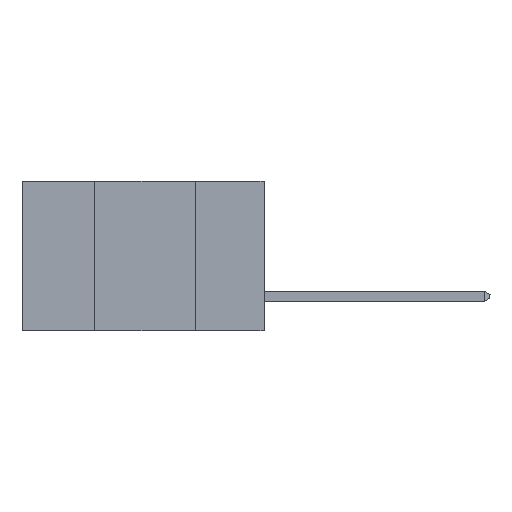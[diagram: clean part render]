
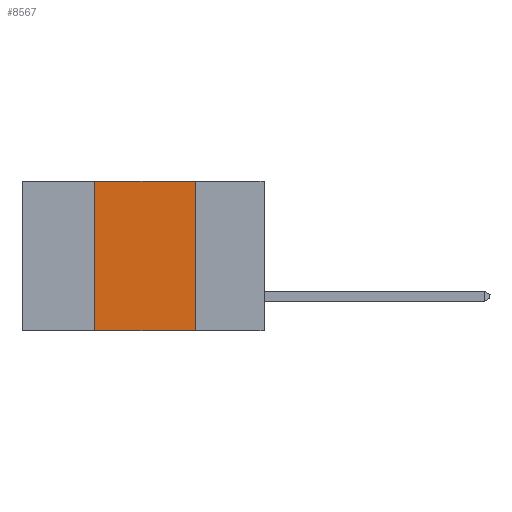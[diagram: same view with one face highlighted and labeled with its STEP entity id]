
A CAD part, left-side view. The second image highlights one B-rep face of the part: STEP entity #8567.
In plain terms, the highlighted planar face has unit normal (-1, 0, 0).
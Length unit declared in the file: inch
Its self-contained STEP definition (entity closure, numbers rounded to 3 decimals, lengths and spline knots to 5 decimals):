
#84 = CARTESIAN_POINT ( 'NONE',  ( 0., 0.42, -0.37 ) ) ;
#148 = CARTESIAN_POINT ( 'NONE',  ( 0., 0.17, -0.37 ) ) ;
#197 = LINE ( 'NONE', #17015, #6263 ) ;
#304 = CARTESIAN_POINT ( 'NONE',  ( 0., 0.6, -0.37 ) ) ;
#472 = LINE ( 'NONE', #304, #10950 ) ;
#909 = CARTESIAN_POINT ( 'NONE',  ( 0., 0.17, 0. ) ) ;
#2550 = EDGE_CURVE ( 'NONE', #17735, #13337, #197, .T. ) ;
#3544 = EDGE_LOOP ( 'NONE', ( #10861, #5936, #5655, #5313 ) ) ;
#4222 = DIRECTION ( 'NONE',  ( 0., -1., 0. ) ) ;
#5313 = ORIENTED_EDGE ( 'NONE', *, *, #16169, .T. ) ;
#5655 = ORIENTED_EDGE ( 'NONE', *, *, #9789, .F. ) ;
#5936 = ORIENTED_EDGE ( 'NONE', *, *, #2550, .F. ) ;
#6263 = VECTOR ( 'NONE', #4222, 39.37008 ) ;
#6573 = FACE_OUTER_BOUND ( 'NONE', #3544, .T. ) ;
#6984 = LINE ( 'NONE', #16964, #15884 ) ;
#7115 = DIRECTION ( 'NONE',  ( 0., 0., -1. ) ) ;
#7387 = DIRECTION ( 'NONE',  ( 1., 0., 0. ) ) ;
#7594 = PLANE ( 'NONE',  #13345 ) ;
#8567 = ADVANCED_FACE ( 'NONE', ( #6573 ), #7594, .F. ) ;
#9500 = VECTOR ( 'NONE', #7115, 39.37008 ) ;
#9789 = EDGE_CURVE ( 'NONE', #9810, #17735, #6984, .T. ) ;
#9810 = VERTEX_POINT ( 'NONE', #84 ) ;
#10308 = DIRECTION ( 'NONE',  ( 0., -1., 0. ) ) ;
#10461 = CARTESIAN_POINT ( 'NONE',  ( 0., 0.6, 0. ) ) ;
#10861 = ORIENTED_EDGE ( 'NONE', *, *, #13388, .F. ) ;
#10950 = VECTOR ( 'NONE', #10308, 39.37008 ) ;
#12739 = VERTEX_POINT ( 'NONE', #148 ) ;
#13337 = VERTEX_POINT ( 'NONE', #909 ) ;
#13345 = AXIS2_PLACEMENT_3D ( 'NONE', #10461, #7387, #14738 ) ;
#13388 = EDGE_CURVE ( 'NONE', #13337, #12739, #14816, .T. ) ;
#14086 = DIRECTION ( 'NONE',  ( 0., 0., 1. ) ) ;
#14738 = DIRECTION ( 'NONE',  ( 0., 0., -1. ) ) ;
#14816 = LINE ( 'NONE', #15371, #9500 ) ;
#15371 = CARTESIAN_POINT ( 'NONE',  ( 0., 0.17, 0. ) ) ;
#15884 = VECTOR ( 'NONE', #14086, 39.37008 ) ;
#16169 = EDGE_CURVE ( 'NONE', #9810, #12739, #472, .T. ) ;
#16295 = CARTESIAN_POINT ( 'NONE',  ( 0., 0.42, 0. ) ) ;
#16964 = CARTESIAN_POINT ( 'NONE',  ( 0., 0.42, 0. ) ) ;
#17015 = CARTESIAN_POINT ( 'NONE',  ( 0., 0.6, 0. ) ) ;
#17735 = VERTEX_POINT ( 'NONE', #16295 ) ;
